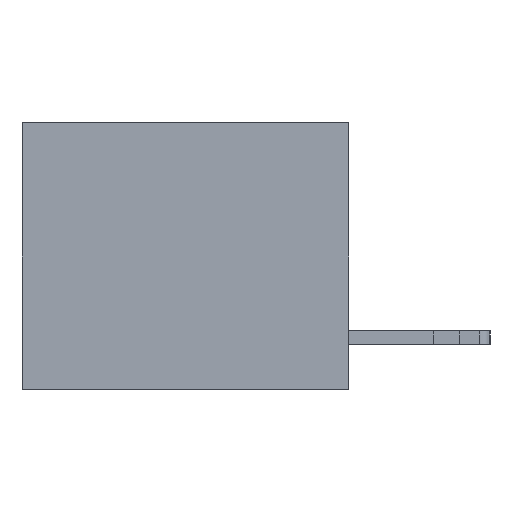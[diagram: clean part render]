
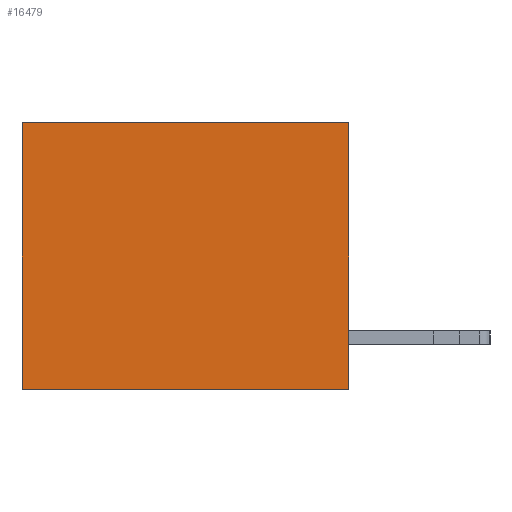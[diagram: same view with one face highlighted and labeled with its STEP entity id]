
A CAD part, left-side view. The second image highlights one B-rep face of the part: STEP entity #16479.
In plain terms, the highlighted planar face has unit normal (-1, 0, 0).
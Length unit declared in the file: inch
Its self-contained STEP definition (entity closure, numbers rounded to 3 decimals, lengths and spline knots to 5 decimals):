
#638 = VERTEX_POINT ( 'NONE', #18472 ) ;
#1550 = VECTOR ( 'NONE', #11511, 39.37008 ) ;
#2110 = CARTESIAN_POINT ( 'NONE',  ( 0.3165, 0., -0.49 ) ) ;
#2339 = VERTEX_POINT ( 'NONE', #16602 ) ;
#2526 = EDGE_CURVE ( 'NONE', #2339, #4673, #5822, .T. ) ;
#2894 = FACE_OUTER_BOUND ( 'NONE', #12899, .T. ) ;
#4387 = EDGE_CURVE ( 'NONE', #20167, #4673, #12229, .T. ) ;
#4565 = DIRECTION ( 'NONE',  ( 0., 0., -1. ) ) ;
#4673 = VERTEX_POINT ( 'NONE', #17226 ) ;
#5822 = LINE ( 'NONE', #14542, #20225 ) ;
#6794 = LINE ( 'NONE', #9851, #21212 ) ;
#7197 = VECTOR ( 'NONE', #4565, 39.37008 ) ;
#9851 = CARTESIAN_POINT ( 'NONE',  ( 0.3165, 0., 0. ) ) ;
#11511 = DIRECTION ( 'NONE',  ( 0., 0., -1. ) ) ;
#11972 = CARTESIAN_POINT ( 'NONE',  ( 0.3165, 0.6, 0. ) ) ;
#12229 = LINE ( 'NONE', #21802, #7197 ) ;
#12899 = EDGE_LOOP ( 'NONE', ( #18464, #15994, #19867, #18103 ) ) ;
#13451 = PLANE ( 'NONE',  #20025 ) ;
#14542 = CARTESIAN_POINT ( 'NONE',  ( 0.3165, 0., -0.49 ) ) ;
#14707 = DIRECTION ( 'NONE',  ( 0., 1., 0. ) ) ;
#15556 = DIRECTION ( 'NONE',  ( 0., 1., 0. ) ) ;
#15994 = ORIENTED_EDGE ( 'NONE', *, *, #2526, .F. ) ;
#16479 = ADVANCED_FACE ( 'NONE', ( #2894 ), #13451, .F. ) ;
#16602 = CARTESIAN_POINT ( 'NONE',  ( 0.3165, 0., -0.49 ) ) ;
#17170 = LINE ( 'NONE', #24366, #1550 ) ;
#17226 = CARTESIAN_POINT ( 'NONE',  ( 0.3165, 0.6, -0.49 ) ) ;
#18103 = ORIENTED_EDGE ( 'NONE', *, *, #22809, .T. ) ;
#18464 = ORIENTED_EDGE ( 'NONE', *, *, #4387, .T. ) ;
#18472 = CARTESIAN_POINT ( 'NONE',  ( 0.3165, 0., 0. ) ) ;
#19237 = EDGE_CURVE ( 'NONE', #638, #2339, #17170, .T. ) ;
#19867 = ORIENTED_EDGE ( 'NONE', *, *, #19237, .F. ) ;
#20025 = AXIS2_PLACEMENT_3D ( 'NONE', #2110, #22817, #21108 ) ;
#20167 = VERTEX_POINT ( 'NONE', #11972 ) ;
#20225 = VECTOR ( 'NONE', #14707, 39.37008 ) ;
#21108 = DIRECTION ( 'NONE',  ( 0., 0., -1. ) ) ;
#21212 = VECTOR ( 'NONE', #15556, 39.37008 ) ;
#21802 = CARTESIAN_POINT ( 'NONE',  ( 0.3165, 0.6, -0.49 ) ) ;
#22809 = EDGE_CURVE ( 'NONE', #638, #20167, #6794, .T. ) ;
#22817 = DIRECTION ( 'NONE',  ( 1., 0., 0. ) ) ;
#24366 = CARTESIAN_POINT ( 'NONE',  ( 0.3165, 0., -0.49 ) ) ;
